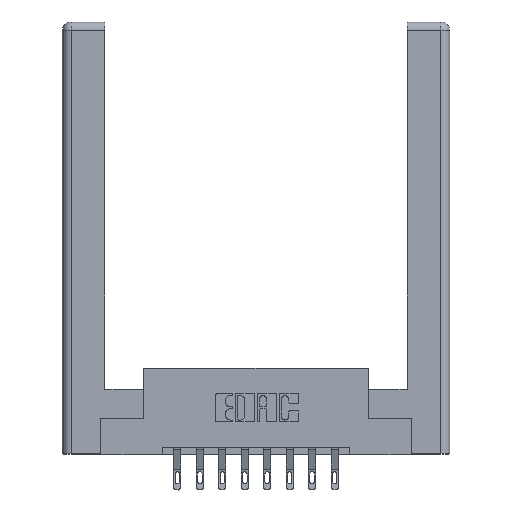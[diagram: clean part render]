
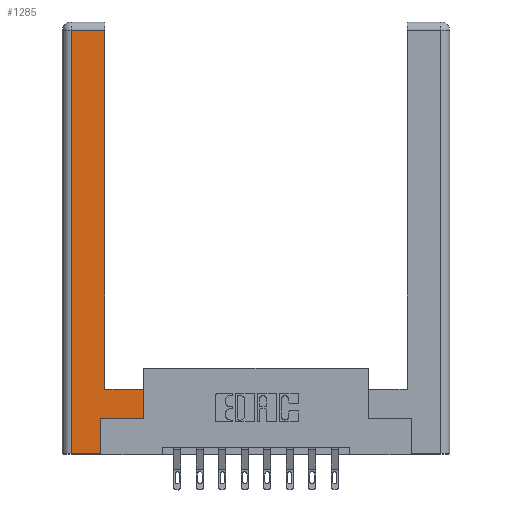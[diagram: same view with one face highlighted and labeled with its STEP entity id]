
A CAD part, top view. The second image highlights one B-rep face of the part: STEP entity #1285.
In plain terms, the highlighted planar face has unit normal (0, 0, 1).
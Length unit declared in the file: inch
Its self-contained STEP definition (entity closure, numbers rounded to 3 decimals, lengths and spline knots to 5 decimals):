
#380 = ORIENTED_EDGE ( 'NONE', *, *, #11999, .T. ) ;
#460 = PLANE ( 'NONE',  #11248 ) ;
#494 = DIRECTION ( 'NONE',  ( -1., 0., 0. ) ) ;
#515 = CARTESIAN_POINT ( 'NONE',  ( 0.565, 0.245, 0. ) ) ;
#610 = ORIENTED_EDGE ( 'NONE', *, *, #3962, .T. ) ;
#626 = DIRECTION ( 'NONE',  ( 0., 1., 0. ) ) ;
#686 = VECTOR ( 'NONE', #626, 39.37008 ) ;
#776 = CARTESIAN_POINT ( 'NONE',  ( 0.0615, 0., 0. ) ) ;
#780 = VERTEX_POINT ( 'NONE', #4451 ) ;
#1063 = VERTEX_POINT ( 'NONE', #776 ) ;
#1285 = ADVANCED_FACE ( 'NONE', ( #9361 ), #460, .F. ) ;
#1317 = CARTESIAN_POINT ( 'NONE',  ( 0.295, 3., 0. ) ) ;
#1437 = VERTEX_POINT ( 'NONE', #13198 ) ;
#1572 = CARTESIAN_POINT ( 'NONE',  ( 0.565, 0.45, 0. ) ) ;
#1808 = VECTOR ( 'NONE', #2260, 39.37008 ) ;
#1820 = VERTEX_POINT ( 'NONE', #8495 ) ;
#1860 = VERTEX_POINT ( 'NONE', #3547 ) ;
#1914 = ORIENTED_EDGE ( 'NONE', *, *, #3504, .T. ) ;
#2043 = CARTESIAN_POINT ( 'NONE',  ( 0.0615, 0., 0. ) ) ;
#2260 = DIRECTION ( 'NONE',  ( 0., 1., 0. ) ) ;
#2328 = ORIENTED_EDGE ( 'NONE', *, *, #5076, .T. ) ;
#2778 = CARTESIAN_POINT ( 'NONE',  ( 0.565, 0.245, 0. ) ) ;
#2890 = DIRECTION ( 'NONE',  ( 1., 0., 0. ) ) ;
#2899 = EDGE_CURVE ( 'NONE', #1860, #12820, #12593, .T. ) ;
#3045 = CARTESIAN_POINT ( 'NONE',  ( 0.0615, 2.94, 0. ) ) ;
#3504 = EDGE_CURVE ( 'NONE', #780, #1063, #10577, .T. ) ;
#3547 = CARTESIAN_POINT ( 'NONE',  ( 0.265, 0.245, 0. ) ) ;
#3661 = LINE ( 'NONE', #7009, #3983 ) ;
#3701 = CARTESIAN_POINT ( 'NONE',  ( 0.265, 0.245, 0. ) ) ;
#3962 = EDGE_CURVE ( 'NONE', #1063, #1820, #3661, .T. ) ;
#3983 = VECTOR ( 'NONE', #2890, 39.37008 ) ;
#4089 = EDGE_LOOP ( 'NONE', ( #380, #8319, #1914, #610, #2328, #6150, #9356, #9498 ) ) ;
#4451 = CARTESIAN_POINT ( 'NONE',  ( 0.0615, 2.94, 0. ) ) ;
#4657 = EDGE_CURVE ( 'NONE', #12366, #12482, #5440, .T. ) ;
#4827 = LINE ( 'NONE', #3045, #10600 ) ;
#5076 = EDGE_CURVE ( 'NONE', #1820, #1860, #10185, .T. ) ;
#5263 = LINE ( 'NONE', #13191, #686 ) ;
#5324 = DIRECTION ( 'NONE',  ( 0., -1., 0. ) ) ;
#5440 = LINE ( 'NONE', #9744, #12479 ) ;
#6012 = CARTESIAN_POINT ( 'NONE',  ( 0.295, 0.45, 0. ) ) ;
#6052 = DIRECTION ( 'NONE',  ( -1., 0., 0. ) ) ;
#6150 = ORIENTED_EDGE ( 'NONE', *, *, #2899, .T. ) ;
#6726 = DIRECTION ( 'NONE',  ( 0., 1., 0. ) ) ;
#7009 = CARTESIAN_POINT ( 'NONE',  ( 0.265, 0., 0. ) ) ;
#7652 = DIRECTION ( 'NONE',  ( -1., 0., 0. ) ) ;
#7786 = CARTESIAN_POINT ( 'NONE',  ( 0., 0., 0. ) ) ;
#8319 = ORIENTED_EDGE ( 'NONE', *, *, #9782, .T. ) ;
#8495 = CARTESIAN_POINT ( 'NONE',  ( 0.265, 0., 0. ) ) ;
#8896 = DIRECTION ( 'NONE',  ( 1., 0., 0. ) ) ;
#9356 = ORIENTED_EDGE ( 'NONE', *, *, #12393, .T. ) ;
#9361 = FACE_OUTER_BOUND ( 'NONE', #4089, .T. ) ;
#9498 = ORIENTED_EDGE ( 'NONE', *, *, #4657, .T. ) ;
#9744 = CARTESIAN_POINT ( 'NONE',  ( 0.295, 0.45, 0. ) ) ;
#9782 = EDGE_CURVE ( 'NONE', #1437, #780, #4827, .T. ) ;
#10185 = LINE ( 'NONE', #3701, #12996 ) ;
#10577 = LINE ( 'NONE', #2043, #11063 ) ;
#10600 = VECTOR ( 'NONE', #6052, 39.37008 ) ;
#10954 = DIRECTION ( 'NONE',  ( 0., 0., -1. ) ) ;
#11063 = VECTOR ( 'NONE', #5324, 39.37008 ) ;
#11248 = AXIS2_PLACEMENT_3D ( 'NONE', #7786, #10954, #494 ) ;
#11526 = LINE ( 'NONE', #1317, #1808 ) ;
#11999 = EDGE_CURVE ( 'NONE', #12482, #1437, #11526, .T. ) ;
#12366 = VERTEX_POINT ( 'NONE', #1572 ) ;
#12393 = EDGE_CURVE ( 'NONE', #12820, #12366, #5263, .T. ) ;
#12479 = VECTOR ( 'NONE', #7652, 39.37008 ) ;
#12482 = VERTEX_POINT ( 'NONE', #6012 ) ;
#12593 = LINE ( 'NONE', #515, #13417 ) ;
#12820 = VERTEX_POINT ( 'NONE', #2778 ) ;
#12996 = VECTOR ( 'NONE', #6726, 39.37008 ) ;
#13191 = CARTESIAN_POINT ( 'NONE',  ( 0.565, 0.45, 0. ) ) ;
#13198 = CARTESIAN_POINT ( 'NONE',  ( 0.295, 2.94, 0. ) ) ;
#13417 = VECTOR ( 'NONE', #8896, 39.37008 ) ;
